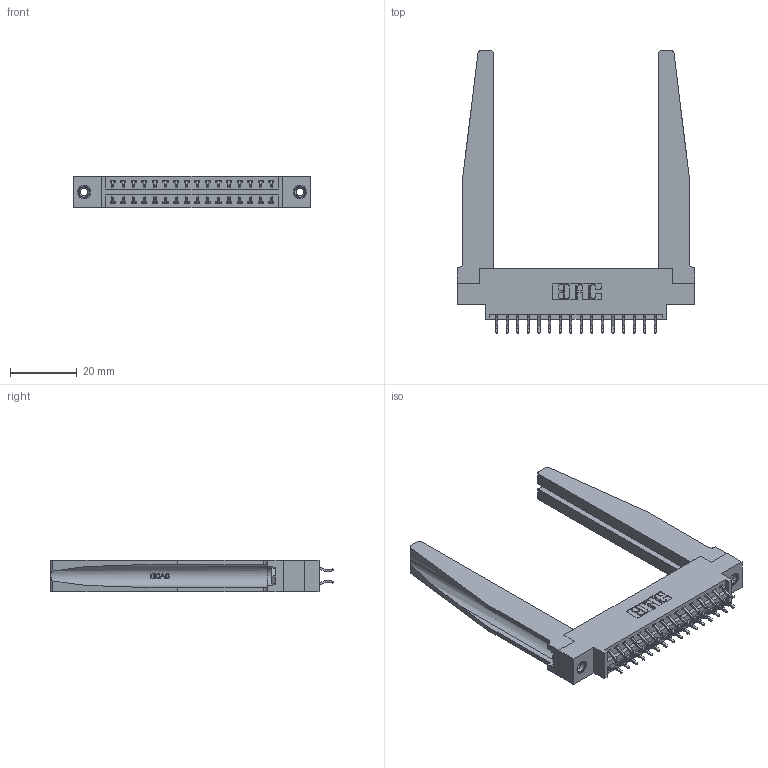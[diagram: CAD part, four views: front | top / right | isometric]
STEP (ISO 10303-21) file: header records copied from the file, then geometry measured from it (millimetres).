
FILE_DESCRIPTION (( 'STEP AP203' ), '1' );
FILE_NAME ('346-032-556-878.STEP', '2022-05-19T18:31:04', ( '' ), ( '' ), 'SwSTEP 2.0', 'SolidWorks 2020', '' );
FILE_SCHEMA (( 'CONFIG_CONTROL_DESIGN' ));
Length unit declared in the file: inch
Products named in the file (5): 345-250-001_345-250-001-102; 345-292-001_556 Tail; 346 Part_0.170 Offset - 0.156 Dia-TH; 346-032-556-878; 346-220-078_345-220-078
Assembly tree (37 placements, depth 2):
  346-032-556-878
    346 Part_0.170 Offset - 0.156 Dia-TH
    345-292-001_556 Tail  x32
    346-220-078_345-220-078  x2
    345-250-001_345-250-001-102  x2
Bounding box: 71.37 x 84.84 x 9.4 mm (x, y, z)
Volume: 13492.8 mm3; surface area: 15363.4 mm2
Topology: 37 solids, 37 shells, 2230 faces, 6521 edges, 4294 vertices
Faces by surface type: plane 1484, cylinder 694, bspline 36, cone 12, torus 4
Entity records: 19458 total; most frequent: CARTESIAN_POINT 4201, ORIENTED_EDGE 3010, DIRECTION 2727, EDGE_CURVE 1505, LINE 1207, VECTOR 1207, VERTEX_POINT 996, AXIS2_PLACEMENT_3D 760
